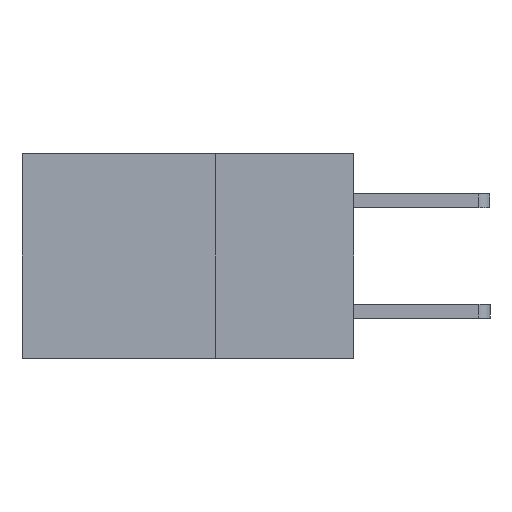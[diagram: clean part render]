
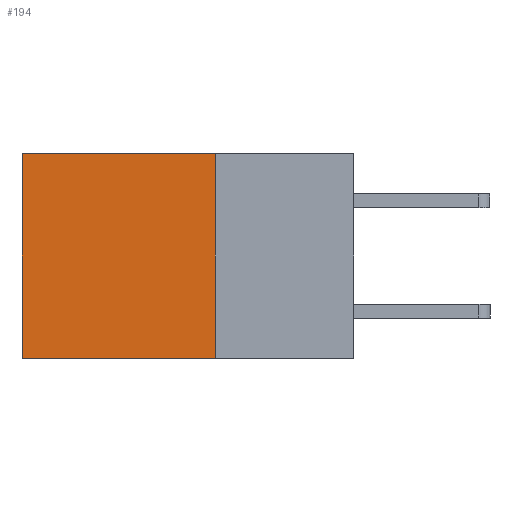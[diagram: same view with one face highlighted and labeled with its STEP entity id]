
A CAD part, left-side view. The second image highlights one B-rep face of the part: STEP entity #194.
In plain terms, the highlighted planar face has unit normal (-1, 0, 0).
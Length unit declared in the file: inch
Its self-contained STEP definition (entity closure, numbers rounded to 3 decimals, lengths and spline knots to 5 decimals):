
#91 = LINE ( 'NONE', #5232, #6801 ) ;
#104 = VERTEX_POINT ( 'NONE', #8062 ) ;
#194 = ADVANCED_FACE ( 'NONE', ( #4715 ), #2216, .F. ) ;
#853 = ORIENTED_EDGE ( 'NONE', *, *, #1293, .T. ) ;
#1293 = EDGE_CURVE ( 'NONE', #4288, #104, #8946, .T. ) ;
#1414 = VECTOR ( 'NONE', #1609, 39.37008 ) ;
#1609 = DIRECTION ( 'NONE',  ( 0., 0., -1. ) ) ;
#1761 = ORIENTED_EDGE ( 'NONE', *, *, #10911, .F. ) ;
#1907 = LINE ( 'NONE', #2988, #4743 ) ;
#2216 = PLANE ( 'NONE',  #4697 ) ;
#2988 = CARTESIAN_POINT ( 'NONE',  ( 0.2875, 0.6, 0. ) ) ;
#3018 = LINE ( 'NONE', #6475, #1414 ) ;
#3367 = VERTEX_POINT ( 'NONE', #7724 ) ;
#4288 = VERTEX_POINT ( 'NONE', #6963 ) ;
#4347 = CARTESIAN_POINT ( 'NONE',  ( 0.2875, 0.25, -0.37 ) ) ;
#4555 = EDGE_CURVE ( 'NONE', #4288, #8805, #3018, .T. ) ;
#4697 = AXIS2_PLACEMENT_3D ( 'NONE', #5798, #5623, #5684 ) ;
#4715 = FACE_OUTER_BOUND ( 'NONE', #6716, .T. ) ;
#4743 = VECTOR ( 'NONE', #5321, 39.37008 ) ;
#5232 = CARTESIAN_POINT ( 'NONE',  ( 0.2875, 0.25, -0.37 ) ) ;
#5321 = DIRECTION ( 'NONE',  ( 0., 0., -1. ) ) ;
#5581 = CARTESIAN_POINT ( 'NONE',  ( 0.2875, 0.25, 0. ) ) ;
#5623 = DIRECTION ( 'NONE',  ( 1., 0., 0. ) ) ;
#5684 = DIRECTION ( 'NONE',  ( 0., 0., -1. ) ) ;
#5798 = CARTESIAN_POINT ( 'NONE',  ( 0.2875, 0.25, 0. ) ) ;
#5951 = EDGE_CURVE ( 'NONE', #104, #3367, #1907, .T. ) ;
#6475 = CARTESIAN_POINT ( 'NONE',  ( 0.2875, 0.25, 0. ) ) ;
#6716 = EDGE_LOOP ( 'NONE', ( #8510, #1761, #8538, #853 ) ) ;
#6801 = VECTOR ( 'NONE', #10582, 39.37008 ) ;
#6963 = CARTESIAN_POINT ( 'NONE',  ( 0.2875, 0.25, 0. ) ) ;
#7724 = CARTESIAN_POINT ( 'NONE',  ( 0.2875, 0.6, -0.37 ) ) ;
#8062 = CARTESIAN_POINT ( 'NONE',  ( 0.2875, 0.6, 0. ) ) ;
#8194 = DIRECTION ( 'NONE',  ( 0., 1., 0. ) ) ;
#8510 = ORIENTED_EDGE ( 'NONE', *, *, #5951, .T. ) ;
#8538 = ORIENTED_EDGE ( 'NONE', *, *, #4555, .F. ) ;
#8805 = VERTEX_POINT ( 'NONE', #4347 ) ;
#8946 = LINE ( 'NONE', #5581, #10063 ) ;
#10063 = VECTOR ( 'NONE', #8194, 39.37008 ) ;
#10582 = DIRECTION ( 'NONE',  ( 0., 1., 0. ) ) ;
#10911 = EDGE_CURVE ( 'NONE', #8805, #3367, #91, .T. ) ;
